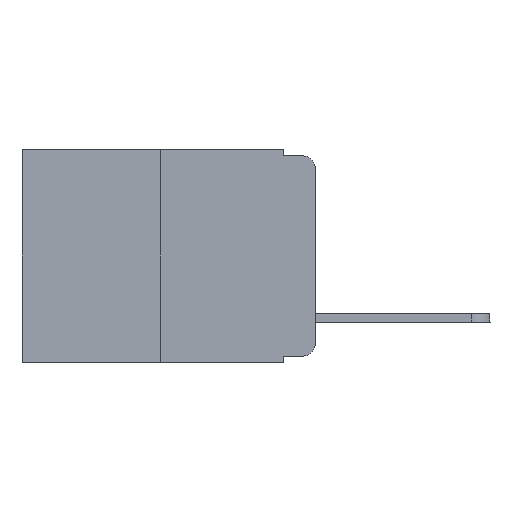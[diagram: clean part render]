
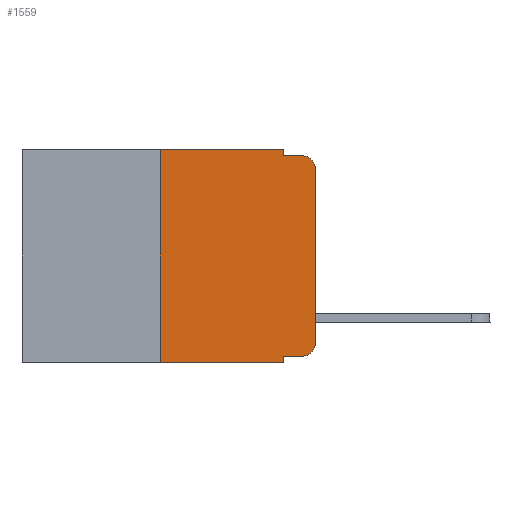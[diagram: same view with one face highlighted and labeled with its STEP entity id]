
A CAD part, left-side view. The second image highlights one B-rep face of the part: STEP entity #1559.
In plain terms, the highlighted planar face has unit normal (-1, 0, 0).
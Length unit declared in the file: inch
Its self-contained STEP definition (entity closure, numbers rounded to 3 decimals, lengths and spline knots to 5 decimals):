
#203 = EDGE_CURVE ( 'NONE', #1750, #20859, #12610, .T. ) ;
#1054 = CARTESIAN_POINT ( 'NONE',  ( 0., 0.051, -0.01 ) ) ;
#1065 = VERTEX_POINT ( 'NONE', #7587 ) ;
#1204 = EDGE_CURVE ( 'NONE', #15622, #11576, #10002, .T. ) ;
#1502 = CARTESIAN_POINT ( 'NONE',  ( 0., 0.051, 0. ) ) ;
#1559 = ADVANCED_FACE ( 'NONE', ( #5543 ), #9328, .F. ) ;
#1656 = ORIENTED_EDGE ( 'NONE', *, *, #23001, .T. ) ;
#1741 = ORIENTED_EDGE ( 'NONE', *, *, #4958, .T. ) ;
#1743 = VECTOR ( 'NONE', #12894, 39.37008 ) ;
#1750 = VERTEX_POINT ( 'NONE', #14770 ) ;
#1992 = ORIENTED_EDGE ( 'NONE', *, *, #20236, .T. ) ;
#2201 = DIRECTION ( 'NONE',  ( 0., 0., -1. ) ) ;
#2459 = LINE ( 'NONE', #12275, #10044 ) ;
#2530 = CARTESIAN_POINT ( 'NONE',  ( 0., 0.02, -0.313 ) ) ;
#2611 = DIRECTION ( 'NONE',  ( 0., 0., -1. ) ) ;
#3460 = LINE ( 'NONE', #13128, #1743 ) ;
#3485 = DIRECTION ( 'NONE',  ( 0., -1., 0. ) ) ;
#3614 = VERTEX_POINT ( 'NONE', #12181 ) ;
#3708 = DIRECTION ( 'NONE',  ( 0., 0., -1. ) ) ;
#4019 = LINE ( 'NONE', #12999, #15181 ) ;
#4094 = VERTEX_POINT ( 'NONE', #1054 ) ;
#4129 = DIRECTION ( 'NONE',  ( 0., 0., 1. ) ) ;
#4211 = CARTESIAN_POINT ( 'NONE',  ( 0., 0.051, 0. ) ) ;
#4703 = CARTESIAN_POINT ( 'NONE',  ( 0., 0.25, 0. ) ) ;
#4914 = CARTESIAN_POINT ( 'NONE',  ( 0., 0.051, -0.343 ) ) ;
#4958 = EDGE_CURVE ( 'NONE', #3614, #1065, #4019, .T. ) ;
#5170 = DIRECTION ( 'NONE',  ( 0., -1., 0. ) ) ;
#5206 = ORIENTED_EDGE ( 'NONE', *, *, #1204, .F. ) ;
#5543 = FACE_OUTER_BOUND ( 'NONE', #21793, .T. ) ;
#5563 = AXIS2_PLACEMENT_3D ( 'NONE', #17508, #11939, #13740 ) ;
#5579 = AXIS2_PLACEMENT_3D ( 'NONE', #12978, #20019, #2201 ) ;
#6129 = ORIENTED_EDGE ( 'NONE', *, *, #18068, .T. ) ;
#6781 = ORIENTED_EDGE ( 'NONE', *, *, #203, .F. ) ;
#7342 = LINE ( 'NONE', #4211, #23057 ) ;
#7587 = CARTESIAN_POINT ( 'NONE',  ( 0., 0., -0.03 ) ) ;
#8569 = CARTESIAN_POINT ( 'NONE',  ( 0., 0.051, 0. ) ) ;
#9328 = PLANE ( 'NONE',  #5579 ) ;
#10002 = LINE ( 'NONE', #13248, #11418 ) ;
#10044 = VECTOR ( 'NONE', #5170, 39.37008 ) ;
#10058 = ORIENTED_EDGE ( 'NONE', *, *, #19623, .F. ) ;
#10902 = AXIS2_PLACEMENT_3D ( 'NONE', #2530, #16812, #2611 ) ;
#11242 = VECTOR ( 'NONE', #3485, 39.37008 ) ;
#11418 = VECTOR ( 'NONE', #20431, 39.37008 ) ;
#11576 = VERTEX_POINT ( 'NONE', #4703 ) ;
#11746 = VERTEX_POINT ( 'NONE', #8569 ) ;
#11881 = VERTEX_POINT ( 'NONE', #21852 ) ;
#11939 = DIRECTION ( 'NONE',  ( -1., 0., 0. ) ) ;
#12090 = CARTESIAN_POINT ( 'NONE',  ( 0., 0.25, -0.343 ) ) ;
#12181 = CARTESIAN_POINT ( 'NONE',  ( 0., 0., -0.313 ) ) ;
#12275 = CARTESIAN_POINT ( 'NONE',  ( 0., 0.051, -0.333 ) ) ;
#12542 = LINE ( 'NONE', #13286, #20365 ) ;
#12610 = LINE ( 'NONE', #1502, #12892 ) ;
#12892 = VECTOR ( 'NONE', #3708, 39.37008 ) ;
#12894 = DIRECTION ( 'NONE',  ( 0., -1., 0. ) ) ;
#12978 = CARTESIAN_POINT ( 'NONE',  ( 0., 0.473, 0. ) ) ;
#12999 = CARTESIAN_POINT ( 'NONE',  ( 0., 0., 0. ) ) ;
#13087 = CIRCLE ( 'NONE', #10902, 0.02 ) ;
#13128 = CARTESIAN_POINT ( 'NONE',  ( 0., 0.473, 0. ) ) ;
#13248 = CARTESIAN_POINT ( 'NONE',  ( 0., 0.25, 0. ) ) ;
#13286 = CARTESIAN_POINT ( 'NONE',  ( 0., 0.473, -0.343 ) ) ;
#13740 = DIRECTION ( 'NONE',  ( 0., 0., -1. ) ) ;
#14127 = ORIENTED_EDGE ( 'NONE', *, *, #19912, .F. ) ;
#14257 = CARTESIAN_POINT ( 'NONE',  ( 0., 0.02, -0.333 ) ) ;
#14696 = EDGE_CURVE ( 'NONE', #11746, #4094, #7342, .T. ) ;
#14770 = CARTESIAN_POINT ( 'NONE',  ( 0., 0.051, -0.333 ) ) ;
#14942 = DIRECTION ( 'NONE',  ( 0., 0., -1. ) ) ;
#15139 = DIRECTION ( 'NONE',  ( 0., -1., 0. ) ) ;
#15181 = VECTOR ( 'NONE', #4129, 39.37008 ) ;
#15460 = ORIENTED_EDGE ( 'NONE', *, *, #22096, .T. ) ;
#15622 = VERTEX_POINT ( 'NONE', #12090 ) ;
#16812 = DIRECTION ( 'NONE',  ( -1., 0., 0. ) ) ;
#16857 = ORIENTED_EDGE ( 'NONE', *, *, #14696, .F. ) ;
#17459 = CARTESIAN_POINT ( 'NONE',  ( 0., 0.051, -0.01 ) ) ;
#17508 = CARTESIAN_POINT ( 'NONE',  ( 0., 0.02, -0.03 ) ) ;
#17885 = VERTEX_POINT ( 'NONE', #14257 ) ;
#18068 = EDGE_CURVE ( 'NONE', #17885, #3614, #13087, .T. ) ;
#19623 = EDGE_CURVE ( 'NONE', #4094, #11881, #21909, .T. ) ;
#19912 = EDGE_CURVE ( 'NONE', #11576, #11746, #3460, .T. ) ;
#20019 = DIRECTION ( 'NONE',  ( 1., 0., 0. ) ) ;
#20236 = EDGE_CURVE ( 'NONE', #1065, #11881, #21025, .T. ) ;
#20365 = VECTOR ( 'NONE', #15139, 39.37008 ) ;
#20431 = DIRECTION ( 'NONE',  ( 0., 0., 1. ) ) ;
#20859 = VERTEX_POINT ( 'NONE', #4914 ) ;
#21025 = CIRCLE ( 'NONE', #5563, 0.02 ) ;
#21793 = EDGE_LOOP ( 'NONE', ( #1741, #1992, #10058, #16857, #14127, #5206, #1656, #6781, #15460, #6129 ) ) ;
#21852 = CARTESIAN_POINT ( 'NONE',  ( 0., 0.02, -0.01 ) ) ;
#21909 = LINE ( 'NONE', #17459, #11242 ) ;
#22096 = EDGE_CURVE ( 'NONE', #1750, #17885, #2459, .T. ) ;
#23001 = EDGE_CURVE ( 'NONE', #15622, #20859, #12542, .T. ) ;
#23057 = VECTOR ( 'NONE', #14942, 39.37008 ) ;
